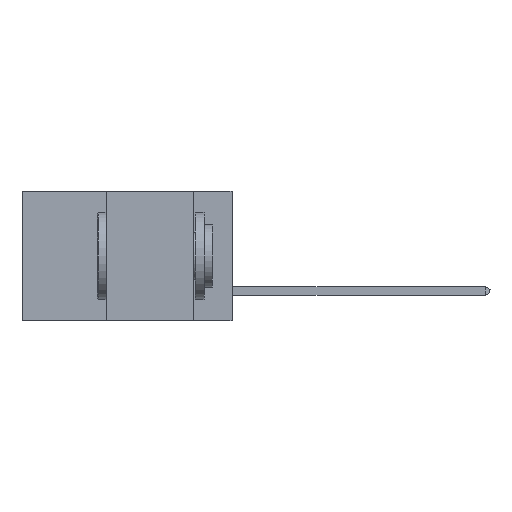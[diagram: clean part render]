
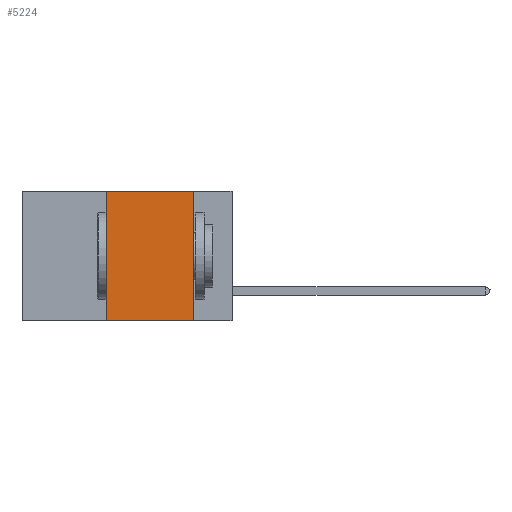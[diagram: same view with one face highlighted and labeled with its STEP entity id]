
A CAD part, left-side view. The second image highlights one B-rep face of the part: STEP entity #5224.
In plain terms, the highlighted planar face has unit normal (-1, 0, 0).
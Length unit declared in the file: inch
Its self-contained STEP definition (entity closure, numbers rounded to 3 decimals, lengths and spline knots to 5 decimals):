
#1861 = PLANE ( 'NONE',  #22420 ) ;
#2378 = CARTESIAN_POINT ( 'NONE',  ( 0., 0.36, 0. ) ) ;
#4805 = CARTESIAN_POINT ( 'NONE',  ( 0., 0.11, 0. ) ) ;
#4869 = VECTOR ( 'NONE', #4958, 39.37008 ) ;
#4958 = DIRECTION ( 'NONE',  ( 0., 0., -1. ) ) ;
#5224 = ADVANCED_FACE ( 'NONE', ( #37852 ), #1861, .F. ) ;
#5978 = DIRECTION ( 'NONE',  ( 0., -1., 0. ) ) ;
#6419 = ORIENTED_EDGE ( 'NONE', *, *, #9381, .F. ) ;
#6578 = EDGE_CURVE ( 'NONE', #32437, #22259, #41485, .T. ) ;
#9205 = LINE ( 'NONE', #4805, #4869 ) ;
#9381 = EDGE_CURVE ( 'NONE', #32437, #17622, #10387, .T. ) ;
#10179 = EDGE_CURVE ( 'NONE', #32135, #22259, #9205, .T. ) ;
#10387 = LINE ( 'NONE', #10993, #26024 ) ;
#10491 = ORIENTED_EDGE ( 'NONE', *, *, #6578, .T. ) ;
#10993 = CARTESIAN_POINT ( 'NONE',  ( 0., 0.36, 0. ) ) ;
#11485 = DIRECTION ( 'NONE',  ( 0., -1., 0. ) ) ;
#14751 = DIRECTION ( 'NONE',  ( 0., 0., 1. ) ) ;
#15897 = DIRECTION ( 'NONE',  ( 1., 0., 0. ) ) ;
#16056 = CARTESIAN_POINT ( 'NONE',  ( 0., 0.6, 0. ) ) ;
#17622 = VERTEX_POINT ( 'NONE', #2378 ) ;
#21064 = ORIENTED_EDGE ( 'NONE', *, *, #41492, .F. ) ;
#22058 = CARTESIAN_POINT ( 'NONE',  ( 0., 0.11, 0. ) ) ;
#22156 = ORIENTED_EDGE ( 'NONE', *, *, #10179, .F. ) ;
#22259 = VERTEX_POINT ( 'NONE', #34706 ) ;
#22420 = AXIS2_PLACEMENT_3D ( 'NONE', #16056, #15897, #26025 ) ;
#22436 = VECTOR ( 'NONE', #11485, 39.37008 ) ;
#24599 = LINE ( 'NONE', #37554, #43552 ) ;
#24764 = CARTESIAN_POINT ( 'NONE',  ( 0., 0.6, -0.37 ) ) ;
#26024 = VECTOR ( 'NONE', #14751, 39.37008 ) ;
#26025 = DIRECTION ( 'NONE',  ( 0., 0., -1. ) ) ;
#32135 = VERTEX_POINT ( 'NONE', #22058 ) ;
#32437 = VERTEX_POINT ( 'NONE', #40331 ) ;
#34706 = CARTESIAN_POINT ( 'NONE',  ( 0., 0.11, -0.37 ) ) ;
#37554 = CARTESIAN_POINT ( 'NONE',  ( 0., 0.6, 0. ) ) ;
#37852 = FACE_OUTER_BOUND ( 'NONE', #44167, .T. ) ;
#40331 = CARTESIAN_POINT ( 'NONE',  ( 0., 0.36, -0.37 ) ) ;
#41485 = LINE ( 'NONE', #24764, #22436 ) ;
#41492 = EDGE_CURVE ( 'NONE', #17622, #32135, #24599, .T. ) ;
#43552 = VECTOR ( 'NONE', #5978, 39.37008 ) ;
#44167 = EDGE_LOOP ( 'NONE', ( #22156, #21064, #6419, #10491 ) ) ;
